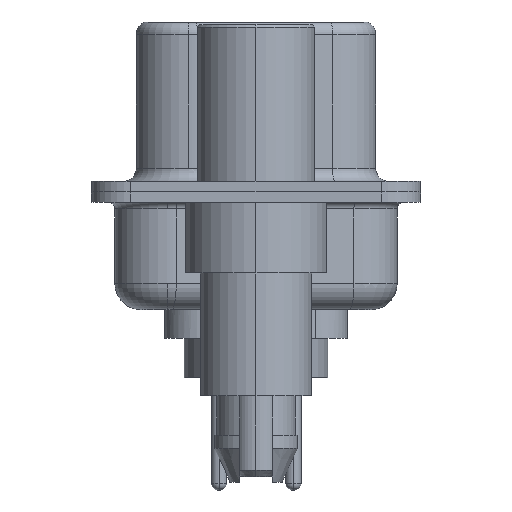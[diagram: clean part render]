
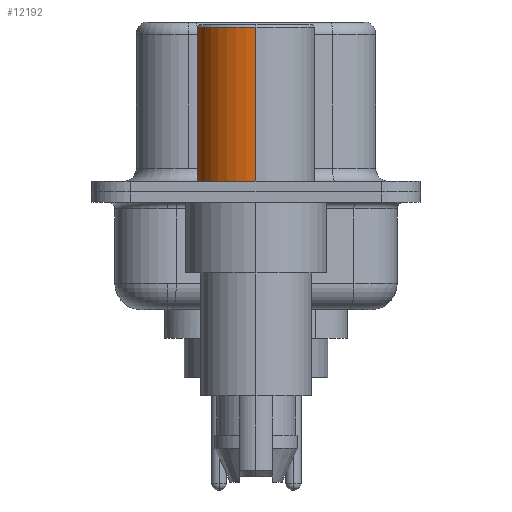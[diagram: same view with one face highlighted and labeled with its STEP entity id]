
A CAD part, left-side view. The second image highlights one B-rep face of the part: STEP entity #12192.
In plain terms, the highlighted cylindrical face has radius 2.25 mm (diameter 4.5 mm), a partial arc.
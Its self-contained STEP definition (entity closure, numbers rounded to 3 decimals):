
#216 = CARTESIAN_POINT ( 'NONE',  ( 2.25, 0., 0.581 ) ) ;
#944 = FACE_OUTER_BOUND ( 'NONE', #16868, .T. ) ;
#1308 = CARTESIAN_POINT ( 'NONE',  ( -2.25, 0., 6.3 ) ) ;
#1826 = DIRECTION ( 'NONE',  ( 0., 0., 1. ) ) ;
#2405 = AXIS2_PLACEMENT_3D ( 'NONE', #14095, #11133, #5279 ) ;
#2449 = CIRCLE ( 'NONE', #17729, 2.25 ) ;
#2646 = ORIENTED_EDGE ( 'NONE', *, *, #14951, .F. ) ;
#2821 = ORIENTED_EDGE ( 'NONE', *, *, #17398, .T. ) ;
#3277 = VERTEX_POINT ( 'NONE', #11587 ) ;
#4630 = DIRECTION ( 'NONE',  ( 0., 0., 1. ) ) ;
#4790 = VERTEX_POINT ( 'NONE', #7043 ) ;
#5146 = ORIENTED_EDGE ( 'NONE', *, *, #12717, .F. ) ;
#5279 = DIRECTION ( 'NONE',  ( 1., 0., 0. ) ) ;
#5513 = VECTOR ( 'NONE', #10963, 1000. ) ;
#5974 = LINE ( 'NONE', #216, #5513 ) ;
#6359 = VERTEX_POINT ( 'NONE', #1308 ) ;
#6554 = CARTESIAN_POINT ( 'NONE',  ( 0., 0., 6.3 ) ) ;
#7043 = CARTESIAN_POINT ( 'NONE',  ( -2.25, 0., 0.4 ) ) ;
#7053 = AXIS2_PLACEMENT_3D ( 'NONE', #10838, #1826, #12336 ) ;
#7634 = CARTESIAN_POINT ( 'NONE',  ( -2.25, 0., 0.581 ) ) ;
#7788 = EDGE_CURVE ( 'NONE', #4790, #6359, #14311, .T. ) ;
#8013 = VERTEX_POINT ( 'NONE', #15451 ) ;
#8073 = DIRECTION ( 'NONE',  ( 1., 0., 0. ) ) ;
#10838 = CARTESIAN_POINT ( 'NONE',  ( 0., 0., 0.4 ) ) ;
#10963 = DIRECTION ( 'NONE',  ( 0., 0., 1. ) ) ;
#11133 = DIRECTION ( 'NONE',  ( 0., 0., 1. ) ) ;
#11587 = CARTESIAN_POINT ( 'NONE',  ( 2.25, 0., 6.3 ) ) ;
#12192 = ADVANCED_FACE ( 'NONE', ( #944 ), #12513, .T. ) ;
#12336 = DIRECTION ( 'NONE',  ( 1., 0., 0. ) ) ;
#12513 = CYLINDRICAL_SURFACE ( 'NONE', #2405, 2.25 ) ;
#12717 = EDGE_CURVE ( 'NONE', #3277, #6359, #2449, .T. ) ;
#13804 = CIRCLE ( 'NONE', #7053, 2.25 ) ;
#14095 = CARTESIAN_POINT ( 'NONE',  ( 0., 0., 0.581 ) ) ;
#14311 = LINE ( 'NONE', #7634, #18481 ) ;
#14951 = EDGE_CURVE ( 'NONE', #8013, #3277, #5974, .T. ) ;
#15451 = CARTESIAN_POINT ( 'NONE',  ( 2.25, 0., 0.4 ) ) ;
#16664 = DIRECTION ( 'NONE',  ( 0., 0., 1. ) ) ;
#16868 = EDGE_LOOP ( 'NONE', ( #2821, #17159, #5146, #2646 ) ) ;
#17159 = ORIENTED_EDGE ( 'NONE', *, *, #7788, .T. ) ;
#17398 = EDGE_CURVE ( 'NONE', #8013, #4790, #13804, .T. ) ;
#17729 = AXIS2_PLACEMENT_3D ( 'NONE', #6554, #16664, #8073 ) ;
#18481 = VECTOR ( 'NONE', #4630, 1000. ) ;
